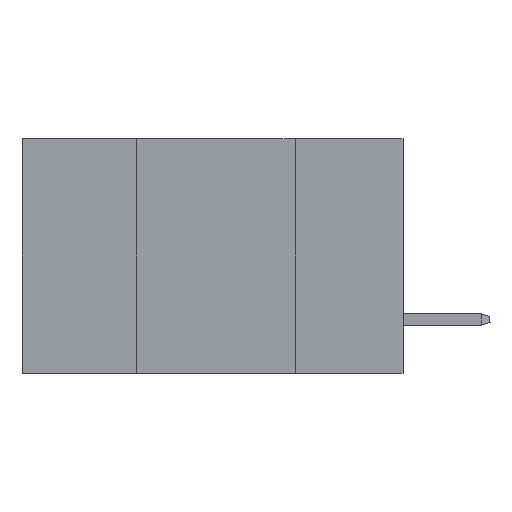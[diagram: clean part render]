
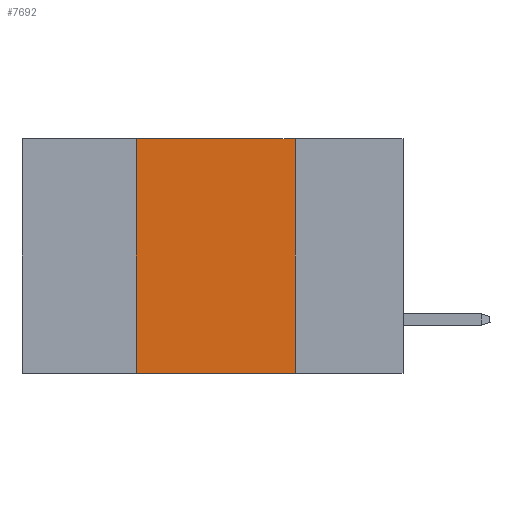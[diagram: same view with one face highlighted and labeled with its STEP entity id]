
A CAD part, left-side view. The second image highlights one B-rep face of the part: STEP entity #7692.
In plain terms, the highlighted planar face has unit normal (-1, 0, 0).
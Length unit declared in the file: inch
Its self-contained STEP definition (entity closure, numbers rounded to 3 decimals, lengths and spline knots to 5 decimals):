
#159 = DIRECTION ( 'NONE',  ( 1., 0., 0. ) ) ;
#347 = ORIENTED_EDGE ( 'NONE', *, *, #17880, .F. ) ;
#442 = LINE ( 'NONE', #7516, #6614 ) ;
#517 = EDGE_CURVE ( 'NONE', #9367, #19108, #11815, .T. ) ;
#1249 = DIRECTION ( 'NONE',  ( 0., -1., 0. ) ) ;
#1705 = FACE_OUTER_BOUND ( 'NONE', #5928, .T. ) ;
#2116 = DIRECTION ( 'NONE',  ( 0., 0., -1. ) ) ;
#2283 = AXIS2_PLACEMENT_3D ( 'NONE', #16599, #159, #7462 ) ;
#2649 = CARTESIAN_POINT ( 'NONE',  ( 0., 0.6, 0. ) ) ;
#2767 = LINE ( 'NONE', #2649, #12832 ) ;
#4694 = ORIENTED_EDGE ( 'NONE', *, *, #517, .T. ) ;
#5308 = CARTESIAN_POINT ( 'NONE',  ( 0., 0.42, -0.37 ) ) ;
#5928 = EDGE_LOOP ( 'NONE', ( #15150, #347, #22127, #4694 ) ) ;
#6614 = VECTOR ( 'NONE', #2116, 39.37008 ) ;
#7462 = DIRECTION ( 'NONE',  ( 0., 0., -1. ) ) ;
#7516 = CARTESIAN_POINT ( 'NONE',  ( 0., 0.17, 0. ) ) ;
#7589 = VERTEX_POINT ( 'NONE', #14557 ) ;
#7692 = ADVANCED_FACE ( 'NONE', ( #1705 ), #9021, .F. ) ;
#9021 = PLANE ( 'NONE',  #2283 ) ;
#9133 = EDGE_CURVE ( 'NONE', #9367, #22065, #10010, .T. ) ;
#9367 = VERTEX_POINT ( 'NONE', #5308 ) ;
#9569 = VECTOR ( 'NONE', #13972, 39.37008 ) ;
#10010 = LINE ( 'NONE', #15881, #9569 ) ;
#11655 = DIRECTION ( 'NONE',  ( 0., -1., 0. ) ) ;
#11706 = VECTOR ( 'NONE', #1249, 39.37008 ) ;
#11815 = LINE ( 'NONE', #17698, #11706 ) ;
#12832 = VECTOR ( 'NONE', #11655, 39.37008 ) ;
#13972 = DIRECTION ( 'NONE',  ( 0., 0., 1. ) ) ;
#14303 = EDGE_CURVE ( 'NONE', #7589, #19108, #442, .T. ) ;
#14557 = CARTESIAN_POINT ( 'NONE',  ( 0., 0.17, 0. ) ) ;
#15150 = ORIENTED_EDGE ( 'NONE', *, *, #14303, .F. ) ;
#15351 = CARTESIAN_POINT ( 'NONE',  ( 0., 0.42, 0. ) ) ;
#15881 = CARTESIAN_POINT ( 'NONE',  ( 0., 0.42, 0. ) ) ;
#16599 = CARTESIAN_POINT ( 'NONE',  ( 0., 0.6, 0. ) ) ;
#17698 = CARTESIAN_POINT ( 'NONE',  ( 0., 0.6, -0.37 ) ) ;
#17880 = EDGE_CURVE ( 'NONE', #22065, #7589, #2767, .T. ) ;
#19108 = VERTEX_POINT ( 'NONE', #20330 ) ;
#20330 = CARTESIAN_POINT ( 'NONE',  ( 0., 0.17, -0.37 ) ) ;
#22065 = VERTEX_POINT ( 'NONE', #15351 ) ;
#22127 = ORIENTED_EDGE ( 'NONE', *, *, #9133, .F. ) ;
